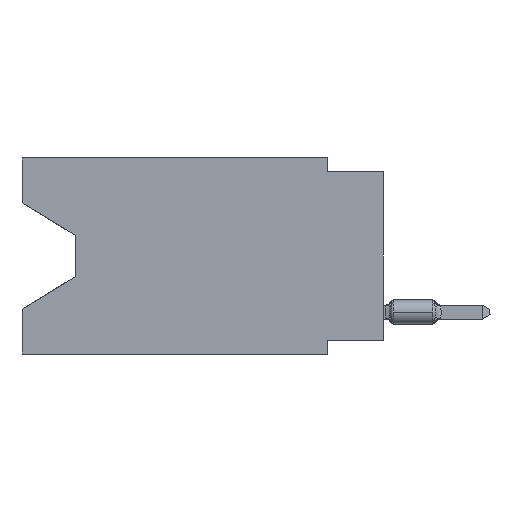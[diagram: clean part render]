
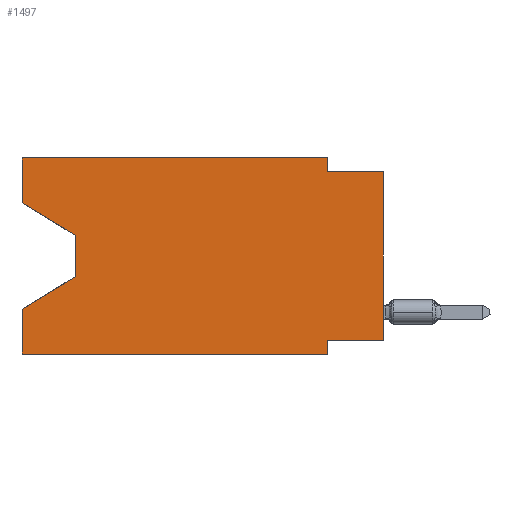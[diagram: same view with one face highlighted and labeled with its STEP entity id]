
A CAD part, left-side view. The second image highlights one B-rep face of the part: STEP entity #1497.
In plain terms, the highlighted planar face has unit normal (-1, 0, 0).
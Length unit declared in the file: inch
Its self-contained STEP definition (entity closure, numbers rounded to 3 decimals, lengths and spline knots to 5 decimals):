
#203 = CARTESIAN_POINT ( 'NONE',  ( 0., 0.645, 0. ) ) ;
#337 = LINE ( 'NONE', #15099, #26776 ) ;
#545 = CARTESIAN_POINT ( 'NONE',  ( 0., 0.55, -0.212 ) ) ;
#820 = LINE ( 'NONE', #13652, #23167 ) ;
#1204 = ORIENTED_EDGE ( 'NONE', *, *, #31939, .F. ) ;
#1497 = ADVANCED_FACE ( 'NONE', ( #27601 ), #15292, .F. ) ;
#1930 = CARTESIAN_POINT ( 'NONE',  ( 0., 0., -0.325 ) ) ;
#1976 = DIRECTION ( 'NONE',  ( 0., -1., 0. ) ) ;
#2025 = DIRECTION ( 'NONE',  ( 0., 0., -1. ) ) ;
#3360 = LINE ( 'NONE', #23164, #16230 ) ;
#3448 = ORIENTED_EDGE ( 'NONE', *, *, #6250, .F. ) ;
#3453 = CARTESIAN_POINT ( 'NONE',  ( 0., 0.1, -0.025 ) ) ;
#3495 = VECTOR ( 'NONE', #15539, 39.37008 ) ;
#3510 = VERTEX_POINT ( 'NONE', #15757 ) ;
#3721 = ORIENTED_EDGE ( 'NONE', *, *, #4816, .T. ) ;
#4816 = EDGE_CURVE ( 'NONE', #13182, #24396, #337, .T. ) ;
#4863 = EDGE_CURVE ( 'NONE', #28622, #17010, #14944, .T. ) ;
#5103 = VERTEX_POINT ( 'NONE', #1930 ) ;
#5192 = DIRECTION ( 'NONE',  ( 0., -0.855, -0.519 ) ) ;
#5378 = DIRECTION ( 'NONE',  ( 0., 0., -1. ) ) ;
#5443 = VECTOR ( 'NONE', #1976, 39.37008 ) ;
#5810 = VECTOR ( 'NONE', #2025, 39.37008 ) ;
#6250 = EDGE_CURVE ( 'NONE', #28622, #20426, #19852, .T. ) ;
#6275 = DIRECTION ( 'NONE',  ( 0., 0., -1. ) ) ;
#6853 = EDGE_CURVE ( 'NONE', #7308, #17010, #25600, .T. ) ;
#7308 = VERTEX_POINT ( 'NONE', #23924 ) ;
#7313 = EDGE_CURVE ( 'NONE', #5103, #25329, #11609, .T. ) ;
#7891 = DIRECTION ( 'NONE',  ( 0., -1., 0. ) ) ;
#8489 = EDGE_CURVE ( 'NONE', #13422, #20426, #20080, .T. ) ;
#9741 = DIRECTION ( 'NONE',  ( 0., -1., 0. ) ) ;
#11220 = EDGE_CURVE ( 'NONE', #14617, #25329, #22823, .T. ) ;
#11221 = CARTESIAN_POINT ( 'NONE',  ( 0., 0.55, -0.138 ) ) ;
#11609 = LINE ( 'NONE', #21642, #23698 ) ;
#12929 = ORIENTED_EDGE ( 'NONE', *, *, #13620, .F. ) ;
#13182 = VERTEX_POINT ( 'NONE', #18571 ) ;
#13249 = EDGE_LOOP ( 'NONE', ( #3721, #28517, #26498, #3448, #25431, #25887, #24106, #15872, #24804, #25463, #12929, #1204 ) ) ;
#13422 = VERTEX_POINT ( 'NONE', #545 ) ;
#13479 = DIRECTION ( 'NONE',  ( 0., 0., 1. ) ) ;
#13620 = EDGE_CURVE ( 'NONE', #26898, #3510, #21769, .T. ) ;
#13652 = CARTESIAN_POINT ( 'NONE',  ( 0., 0.645, 0. ) ) ;
#13860 = VECTOR ( 'NONE', #9741, 39.37008 ) ;
#14617 = VERTEX_POINT ( 'NONE', #3453 ) ;
#14944 = LINE ( 'NONE', #31945, #13860 ) ;
#15099 = CARTESIAN_POINT ( 'NONE',  ( 0., 0.645, -0.08025 ) ) ;
#15292 = PLANE ( 'NONE',  #31708 ) ;
#15539 = DIRECTION ( 'NONE',  ( 0., 0.855, -0.519 ) ) ;
#15757 = CARTESIAN_POINT ( 'NONE',  ( 0., 0.1, 0. ) ) ;
#15872 = ORIENTED_EDGE ( 'NONE', *, *, #7313, .T. ) ;
#15981 = EDGE_CURVE ( 'NONE', #24396, #13422, #24261, .T. ) ;
#16230 = VECTOR ( 'NONE', #30603, 39.37008 ) ;
#17010 = VERTEX_POINT ( 'NONE', #28010 ) ;
#17951 = LINE ( 'NONE', #28177, #24830 ) ;
#18519 = VECTOR ( 'NONE', #29748, 39.37008 ) ;
#18571 = CARTESIAN_POINT ( 'NONE',  ( 0., 0.645, -0.08025 ) ) ;
#19852 = LINE ( 'NONE', #25523, #18519 ) ;
#20080 = LINE ( 'NONE', #29974, #3495 ) ;
#20426 = VERTEX_POINT ( 'NONE', #26986 ) ;
#21642 = CARTESIAN_POINT ( 'NONE',  ( 0., 0., 0. ) ) ;
#21769 = LINE ( 'NONE', #24527, #5443 ) ;
#22823 = LINE ( 'NONE', #27509, #31843 ) ;
#23164 = CARTESIAN_POINT ( 'NONE',  ( 0., 0., -0.325 ) ) ;
#23167 = VECTOR ( 'NONE', #13479, 39.37008 ) ;
#23326 = CARTESIAN_POINT ( 'NONE',  ( 0., 0.1, -0.35 ) ) ;
#23698 = VECTOR ( 'NONE', #29255, 39.37008 ) ;
#23924 = CARTESIAN_POINT ( 'NONE',  ( 0., 0.1, -0.325 ) ) ;
#24106 = ORIENTED_EDGE ( 'NONE', *, *, #31310, .F. ) ;
#24261 = LINE ( 'NONE', #31385, #5810 ) ;
#24396 = VERTEX_POINT ( 'NONE', #11221 ) ;
#24527 = CARTESIAN_POINT ( 'NONE',  ( 0., 0.645, 0. ) ) ;
#24629 = CARTESIAN_POINT ( 'NONE',  ( 0., 0.645, -0.35 ) ) ;
#24804 = ORIENTED_EDGE ( 'NONE', *, *, #11220, .F. ) ;
#24830 = VECTOR ( 'NONE', #27837, 39.37008 ) ;
#25178 = DIRECTION ( 'NONE',  ( 1., 0., 0. ) ) ;
#25221 = EDGE_CURVE ( 'NONE', #3510, #14617, #17951, .T. ) ;
#25329 = VERTEX_POINT ( 'NONE', #30285 ) ;
#25431 = ORIENTED_EDGE ( 'NONE', *, *, #4863, .T. ) ;
#25463 = ORIENTED_EDGE ( 'NONE', *, *, #25221, .F. ) ;
#25523 = CARTESIAN_POINT ( 'NONE',  ( 0., 0.645, 0. ) ) ;
#25600 = LINE ( 'NONE', #23326, #31479 ) ;
#25887 = ORIENTED_EDGE ( 'NONE', *, *, #6853, .F. ) ;
#26498 = ORIENTED_EDGE ( 'NONE', *, *, #8489, .T. ) ;
#26776 = VECTOR ( 'NONE', #5192, 39.37008 ) ;
#26898 = VERTEX_POINT ( 'NONE', #27082 ) ;
#26986 = CARTESIAN_POINT ( 'NONE',  ( 0., 0.645, -0.26975 ) ) ;
#27082 = CARTESIAN_POINT ( 'NONE',  ( 0., 0.645, 0. ) ) ;
#27509 = CARTESIAN_POINT ( 'NONE',  ( 0., 0., -0.025 ) ) ;
#27601 = FACE_OUTER_BOUND ( 'NONE', #13249, .T. ) ;
#27837 = DIRECTION ( 'NONE',  ( 0., 0., -1. ) ) ;
#28010 = CARTESIAN_POINT ( 'NONE',  ( 0., 0.1, -0.35 ) ) ;
#28177 = CARTESIAN_POINT ( 'NONE',  ( 0., 0.1, 0. ) ) ;
#28517 = ORIENTED_EDGE ( 'NONE', *, *, #15981, .T. ) ;
#28622 = VERTEX_POINT ( 'NONE', #24629 ) ;
#29255 = DIRECTION ( 'NONE',  ( 0., 0., 1. ) ) ;
#29748 = DIRECTION ( 'NONE',  ( 0., 0., 1. ) ) ;
#29974 = CARTESIAN_POINT ( 'NONE',  ( 0., 0.55, -0.212 ) ) ;
#30285 = CARTESIAN_POINT ( 'NONE',  ( 0., 0., -0.025 ) ) ;
#30603 = DIRECTION ( 'NONE',  ( 0., 1., 0. ) ) ;
#31310 = EDGE_CURVE ( 'NONE', #5103, #7308, #3360, .T. ) ;
#31385 = CARTESIAN_POINT ( 'NONE',  ( 0., 0.55, -0.138 ) ) ;
#31479 = VECTOR ( 'NONE', #6275, 39.37008 ) ;
#31708 = AXIS2_PLACEMENT_3D ( 'NONE', #203, #25178, #5378 ) ;
#31843 = VECTOR ( 'NONE', #7891, 39.37008 ) ;
#31939 = EDGE_CURVE ( 'NONE', #13182, #26898, #820, .T. ) ;
#31945 = CARTESIAN_POINT ( 'NONE',  ( 0., 0.645, -0.35 ) ) ;
